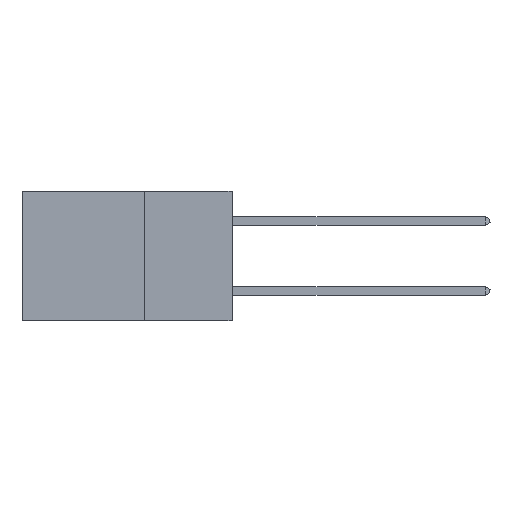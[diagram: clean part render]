
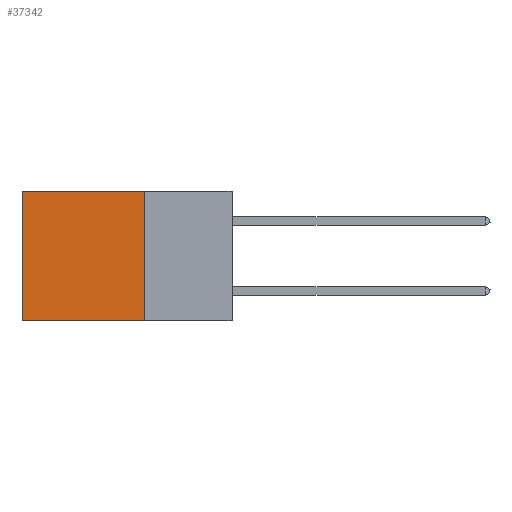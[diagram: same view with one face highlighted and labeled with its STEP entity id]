
A CAD part, left-side view. The second image highlights one B-rep face of the part: STEP entity #37342.
In plain terms, the highlighted planar face has unit normal (-1, 0, 0).
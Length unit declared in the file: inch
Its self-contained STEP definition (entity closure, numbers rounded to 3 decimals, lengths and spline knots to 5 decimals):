
#447 = EDGE_LOOP ( 'NONE', ( #35001, #26506, #11926, #10689 ) ) ;
#1411 = LINE ( 'NONE', #14157, #11923 ) ;
#1484 = VECTOR ( 'NONE', #3534, 39.37008 ) ;
#2373 = VERTEX_POINT ( 'NONE', #34947 ) ;
#3055 = VECTOR ( 'NONE', #8420, 39.37008 ) ;
#3534 = DIRECTION ( 'NONE',  ( 0., 1., 0. ) ) ;
#6036 = VERTEX_POINT ( 'NONE', #32477 ) ;
#7809 = FACE_OUTER_BOUND ( 'NONE', #447, .T. ) ;
#8420 = DIRECTION ( 'NONE',  ( 0., 0., -1. ) ) ;
#9857 = LINE ( 'NONE', #20371, #1484 ) ;
#10635 = VERTEX_POINT ( 'NONE', #41913 ) ;
#10689 = ORIENTED_EDGE ( 'NONE', *, *, #12416, .T. ) ;
#11923 = VECTOR ( 'NONE', #17670, 39.37008 ) ;
#11926 = ORIENTED_EDGE ( 'NONE', *, *, #35115, .F. ) ;
#12416 = EDGE_CURVE ( 'NONE', #2373, #10635, #1411, .T. ) ;
#12507 = LINE ( 'NONE', #18676, #3055 ) ;
#14157 = CARTESIAN_POINT ( 'NONE',  ( 0.2875, 0.25, 0. ) ) ;
#15456 = DIRECTION ( 'NONE',  ( 1., 0., 0. ) ) ;
#15826 = VERTEX_POINT ( 'NONE', #18648 ) ;
#17670 = DIRECTION ( 'NONE',  ( 0., 1., 0. ) ) ;
#18648 = CARTESIAN_POINT ( 'NONE',  ( 0.2875, 0.25, -0.37 ) ) ;
#18676 = CARTESIAN_POINT ( 'NONE',  ( 0.2875, 0.6, 0. ) ) ;
#19449 = EDGE_CURVE ( 'NONE', #10635, #6036, #12507, .T. ) ;
#20206 = CARTESIAN_POINT ( 'NONE',  ( 0.2875, 0.25, 0. ) ) ;
#20371 = CARTESIAN_POINT ( 'NONE',  ( 0.2875, 0.25, -0.37 ) ) ;
#25946 = CARTESIAN_POINT ( 'NONE',  ( 0.2875, 0.25, 0. ) ) ;
#26506 = ORIENTED_EDGE ( 'NONE', *, *, #37568, .F. ) ;
#27394 = VECTOR ( 'NONE', #30281, 39.37008 ) ;
#30281 = DIRECTION ( 'NONE',  ( 0., 0., -1. ) ) ;
#32117 = PLANE ( 'NONE',  #39001 ) ;
#32477 = CARTESIAN_POINT ( 'NONE',  ( 0.2875, 0.6, -0.37 ) ) ;
#34947 = CARTESIAN_POINT ( 'NONE',  ( 0.2875, 0.25, 0. ) ) ;
#35001 = ORIENTED_EDGE ( 'NONE', *, *, #19449, .T. ) ;
#35115 = EDGE_CURVE ( 'NONE', #2373, #15826, #35203, .T. ) ;
#35203 = LINE ( 'NONE', #20206, #27394 ) ;
#37342 = ADVANCED_FACE ( 'NONE', ( #7809 ), #32117, .F. ) ;
#37568 = EDGE_CURVE ( 'NONE', #15826, #6036, #9857, .T. ) ;
#39001 = AXIS2_PLACEMENT_3D ( 'NONE', #25946, #15456, #42349 ) ;
#41913 = CARTESIAN_POINT ( 'NONE',  ( 0.2875, 0.6, 0. ) ) ;
#42349 = DIRECTION ( 'NONE',  ( 0., 0., -1. ) ) ;
